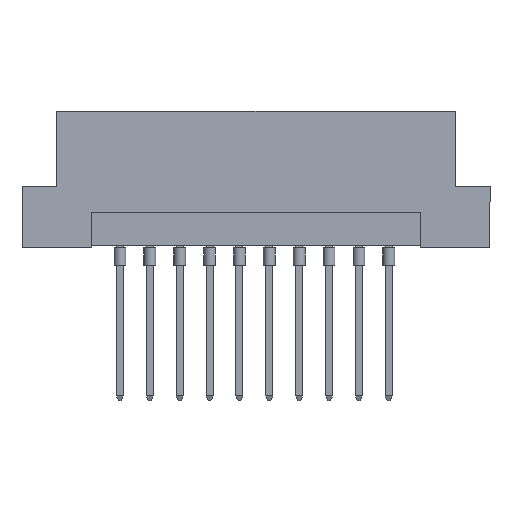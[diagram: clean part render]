
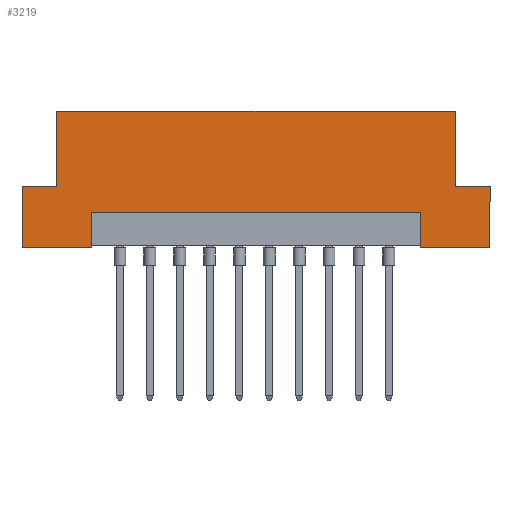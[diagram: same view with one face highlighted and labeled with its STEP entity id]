
A CAD part, front view. The second image highlights one B-rep face of the part: STEP entity #3219.
In plain terms, the highlighted planar face has unit normal (0, -1, 0).
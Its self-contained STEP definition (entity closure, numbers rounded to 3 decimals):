
#157 = DIRECTION ( 'NONE',  ( 1., 0., 0. ) ) ;
#172 = DIRECTION ( 'NONE',  ( 0., 0., 1. ) ) ;
#209 = VERTEX_POINT ( 'NONE', #3205 ) ;
#242 = DIRECTION ( 'NONE',  ( -1., 0., 0. ) ) ;
#339 = VECTOR ( 'NONE', #1164, 1000. ) ;
#545 = CARTESIAN_POINT ( 'NONE',  ( -14., -4.3, 0.2 ) ) ;
#571 = VERTEX_POINT ( 'NONE', #4717 ) ;
#601 = DIRECTION ( 'NONE',  ( 0., 0., -1. ) ) ;
#616 = VECTOR ( 'NONE', #3031, 1000. ) ;
#664 = LINE ( 'NONE', #5226, #339 ) ;
#684 = CARTESIAN_POINT ( 'NONE',  ( 16.94, -4.3, 5.2 ) ) ;
#879 = VERTEX_POINT ( 'NONE', #684 ) ;
#882 = CARTESIAN_POINT ( 'NONE',  ( 16.94, -4.3, 11.6 ) ) ;
#888 = CARTESIAN_POINT ( 'NONE',  ( -16.94, -4.3, 5.2 ) ) ;
#953 = LINE ( 'NONE', #545, #4445 ) ;
#986 = EDGE_CURVE ( 'NONE', #2269, #1827, #953, .T. ) ;
#987 = CARTESIAN_POINT ( 'NONE',  ( -19.9, -4.3, 5.2 ) ) ;
#1025 = VECTOR ( 'NONE', #5193, 1000. ) ;
#1091 = ORIENTED_EDGE ( 'NONE', *, *, #1762, .F. ) ;
#1124 = VECTOR ( 'NONE', #3804, 1000. ) ;
#1143 = AXIS2_PLACEMENT_3D ( 'NONE', #2226, #1840, #242 ) ;
#1164 = DIRECTION ( 'NONE',  ( 1., 0., 0. ) ) ;
#1198 = LINE ( 'NONE', #4463, #1969 ) ;
#1241 = EDGE_CURVE ( 'NONE', #209, #3399, #1198, .T. ) ;
#1334 = ORIENTED_EDGE ( 'NONE', *, *, #4080, .T. ) ;
#1372 = LINE ( 'NONE', #987, #1374 ) ;
#1374 = VECTOR ( 'NONE', #2947, 1000. ) ;
#1402 = EDGE_LOOP ( 'NONE', ( #1334, #4355, #4699, #2122, #2485, #5184, #4734, #2110, #1091, #5176, #2941, #5100 ) ) ;
#1407 = FACE_OUTER_BOUND ( 'NONE', #1402, .T. ) ;
#1592 = EDGE_CURVE ( 'NONE', #2790, #3399, #4490, .T. ) ;
#1710 = LINE ( 'NONE', #4964, #1124 ) ;
#1762 = EDGE_CURVE ( 'NONE', #571, #3571, #1372, .T. ) ;
#1827 = VERTEX_POINT ( 'NONE', #2613 ) ;
#1829 = VECTOR ( 'NONE', #172, 1000. ) ;
#1840 = DIRECTION ( 'NONE',  ( 0., 1., 0. ) ) ;
#1857 = DIRECTION ( 'NONE',  ( 0., 0., -1. ) ) ;
#1953 = EDGE_CURVE ( 'NONE', #4246, #2225, #664, .T. ) ;
#1969 = VECTOR ( 'NONE', #1857, 1000. ) ;
#1974 = VECTOR ( 'NONE', #4035, 1000. ) ;
#2042 = DIRECTION ( 'NONE',  ( 1., 0., 0. ) ) ;
#2110 = ORIENTED_EDGE ( 'NONE', *, *, #2825, .F. ) ;
#2119 = CARTESIAN_POINT ( 'NONE',  ( -14., -4.3, 3. ) ) ;
#2122 = ORIENTED_EDGE ( 'NONE', *, *, #1241, .F. ) ;
#2225 = VERTEX_POINT ( 'NONE', #882 ) ;
#2226 = CARTESIAN_POINT ( 'NONE',  ( 19.9, -4.3, 11.6 ) ) ;
#2233 = CARTESIAN_POINT ( 'NONE',  ( 14., -4.3, 0. ) ) ;
#2248 = LINE ( 'NONE', #4229, #2805 ) ;
#2269 = VERTEX_POINT ( 'NONE', #4309 ) ;
#2277 = PLANE ( 'NONE',  #1143 ) ;
#2378 = LINE ( 'NONE', #4858, #3422 ) ;
#2485 = ORIENTED_EDGE ( 'NONE', *, *, #3661, .F. ) ;
#2613 = CARTESIAN_POINT ( 'NONE',  ( -14., -4.3, 0. ) ) ;
#2734 = CARTESIAN_POINT ( 'NONE',  ( 19.9, -4.3, 0. ) ) ;
#2790 = VERTEX_POINT ( 'NONE', #2233 ) ;
#2805 = VECTOR ( 'NONE', #157, 1000. ) ;
#2825 = EDGE_CURVE ( 'NONE', #3571, #4246, #3926, .T. ) ;
#2941 = ORIENTED_EDGE ( 'NONE', *, *, #5296, .T. ) ;
#2947 = DIRECTION ( 'NONE',  ( 1., 0., 0. ) ) ;
#2962 = CARTESIAN_POINT ( 'NONE',  ( 14., -4.3, 3. ) ) ;
#3031 = DIRECTION ( 'NONE',  ( 0., 0., 1. ) ) ;
#3126 = CARTESIAN_POINT ( 'NONE',  ( -19.9, -4.3, 11.6 ) ) ;
#3205 = CARTESIAN_POINT ( 'NONE',  ( 19.9, -4.3, 5.2 ) ) ;
#3219 = ADVANCED_FACE ( 'NONE', ( #1407 ), #2277, .F. ) ;
#3292 = EDGE_CURVE ( 'NONE', #879, #2225, #5104, .T. ) ;
#3397 = DIRECTION ( 'NONE',  ( 1., 0., 0. ) ) ;
#3399 = VERTEX_POINT ( 'NONE', #4375 ) ;
#3422 = VECTOR ( 'NONE', #2042, 1000. ) ;
#3450 = CARTESIAN_POINT ( 'NONE',  ( -16.94, -4.3, 5.2 ) ) ;
#3451 = LINE ( 'NONE', #3126, #1025 ) ;
#3571 = VERTEX_POINT ( 'NONE', #888 ) ;
#3661 = EDGE_CURVE ( 'NONE', #879, #209, #2248, .T. ) ;
#3705 = VERTEX_POINT ( 'NONE', #4417 ) ;
#3804 = DIRECTION ( 'NONE',  ( 0., 0., 1. ) ) ;
#3816 = LINE ( 'NONE', #2119, #3839 ) ;
#3839 = VECTOR ( 'NONE', #3397, 1000. ) ;
#3926 = LINE ( 'NONE', #3450, #1829 ) ;
#3984 = CARTESIAN_POINT ( 'NONE',  ( -16.94, -4.3, 11.6 ) ) ;
#4035 = DIRECTION ( 'NONE',  ( 1., 0., 0. ) ) ;
#4080 = EDGE_CURVE ( 'NONE', #2269, #4112, #3816, .T. ) ;
#4112 = VERTEX_POINT ( 'NONE', #2962 ) ;
#4139 = EDGE_CURVE ( 'NONE', #571, #3705, #3451, .T. ) ;
#4229 = CARTESIAN_POINT ( 'NONE',  ( 19.9, -4.3, 5.2 ) ) ;
#4246 = VERTEX_POINT ( 'NONE', #3984 ) ;
#4309 = CARTESIAN_POINT ( 'NONE',  ( -14., -4.3, 3. ) ) ;
#4355 = ORIENTED_EDGE ( 'NONE', *, *, #4961, .F. ) ;
#4375 = CARTESIAN_POINT ( 'NONE',  ( 19.9, -4.3, 0. ) ) ;
#4417 = CARTESIAN_POINT ( 'NONE',  ( -19.9, -4.3, 0. ) ) ;
#4445 = VECTOR ( 'NONE', #601, 1000. ) ;
#4463 = CARTESIAN_POINT ( 'NONE',  ( 19.9, -4.3, 11.6 ) ) ;
#4490 = LINE ( 'NONE', #2734, #1974 ) ;
#4699 = ORIENTED_EDGE ( 'NONE', *, *, #1592, .T. ) ;
#4710 = CARTESIAN_POINT ( 'NONE',  ( 16.94, -4.3, 5.2 ) ) ;
#4717 = CARTESIAN_POINT ( 'NONE',  ( -19.9, -4.3, 5.2 ) ) ;
#4734 = ORIENTED_EDGE ( 'NONE', *, *, #1953, .F. ) ;
#4858 = CARTESIAN_POINT ( 'NONE',  ( 19.9, -4.3, 0. ) ) ;
#4961 = EDGE_CURVE ( 'NONE', #2790, #4112, #1710, .T. ) ;
#4964 = CARTESIAN_POINT ( 'NONE',  ( 14., -4.3, 0.2 ) ) ;
#5100 = ORIENTED_EDGE ( 'NONE', *, *, #986, .F. ) ;
#5104 = LINE ( 'NONE', #4710, #616 ) ;
#5176 = ORIENTED_EDGE ( 'NONE', *, *, #4139, .T. ) ;
#5184 = ORIENTED_EDGE ( 'NONE', *, *, #3292, .T. ) ;
#5193 = DIRECTION ( 'NONE',  ( 0., 0., -1. ) ) ;
#5226 = CARTESIAN_POINT ( 'NONE',  ( 19.9, -4.3, 11.6 ) ) ;
#5296 = EDGE_CURVE ( 'NONE', #3705, #1827, #2378, .T. ) ;
